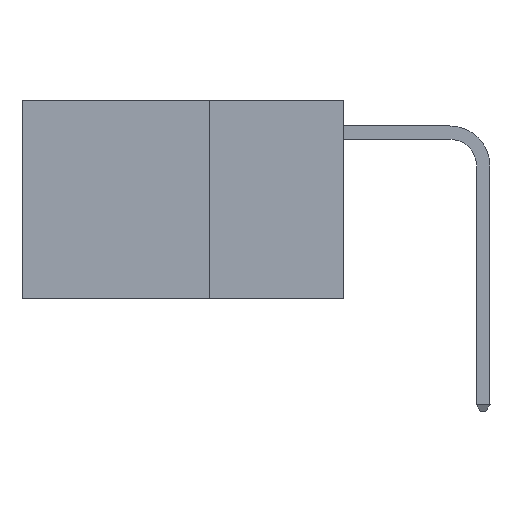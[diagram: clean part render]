
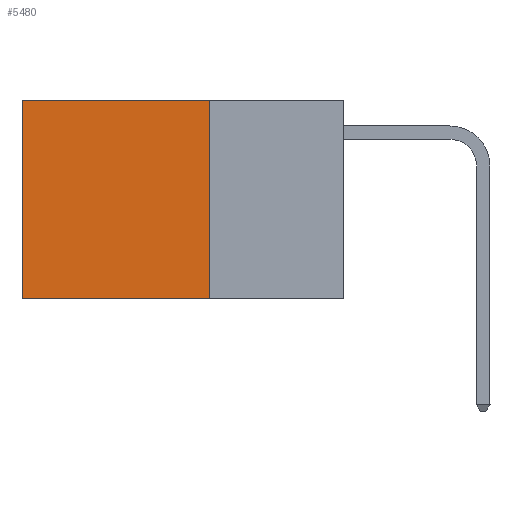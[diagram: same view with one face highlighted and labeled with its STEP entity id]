
A CAD part, left-side view. The second image highlights one B-rep face of the part: STEP entity #5480.
In plain terms, the highlighted planar face has unit normal (-1, 0, 0).
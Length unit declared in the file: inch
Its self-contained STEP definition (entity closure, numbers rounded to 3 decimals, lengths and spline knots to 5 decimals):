
#36 = DIRECTION ( 'NONE',  ( 0., 0., -1. ) ) ;
#154 = DIRECTION ( 'NONE',  ( 1., 0., 0. ) ) ;
#288 = CARTESIAN_POINT ( 'NONE',  ( 0.2625, 0.6, 0. ) ) ;
#402 = VERTEX_POINT ( 'NONE', #11299 ) ;
#487 = EDGE_CURVE ( 'NONE', #6970, #2752, #10767, .T. ) ;
#626 = ORIENTED_EDGE ( 'NONE', *, *, #5296, .F. ) ;
#1123 = ORIENTED_EDGE ( 'NONE', *, *, #6794, .F. ) ;
#2195 = CARTESIAN_POINT ( 'NONE',  ( 0.2625, 0.25, 0. ) ) ;
#2482 = CARTESIAN_POINT ( 'NONE',  ( 0.2625, 0.25, 0. ) ) ;
#2663 = FACE_OUTER_BOUND ( 'NONE', #4842, .T. ) ;
#2690 = VECTOR ( 'NONE', #9444, 39.37008 ) ;
#2752 = VERTEX_POINT ( 'NONE', #288 ) ;
#3452 = VECTOR ( 'NONE', #6245, 39.37008 ) ;
#3512 = AXIS2_PLACEMENT_3D ( 'NONE', #12744, #154, #7525 ) ;
#4135 = CARTESIAN_POINT ( 'NONE',  ( 0.2625, 0.6, 0. ) ) ;
#4176 = ORIENTED_EDGE ( 'NONE', *, *, #13438, .T. ) ;
#4400 = VERTEX_POINT ( 'NONE', #6271 ) ;
#4842 = EDGE_LOOP ( 'NONE', ( #4176, #626, #1123, #9926 ) ) ;
#5296 = EDGE_CURVE ( 'NONE', #402, #4400, #7436, .T. ) ;
#5407 = PLANE ( 'NONE',  #3512 ) ;
#5480 = ADVANCED_FACE ( 'NONE', ( #2663 ), #5407, .F. ) ;
#6245 = DIRECTION ( 'NONE',  ( 0., 0., -1. ) ) ;
#6271 = CARTESIAN_POINT ( 'NONE',  ( 0.2625, 0.6, -0.37 ) ) ;
#6794 = EDGE_CURVE ( 'NONE', #6970, #402, #7554, .T. ) ;
#6970 = VERTEX_POINT ( 'NONE', #2482 ) ;
#7436 = LINE ( 'NONE', #9280, #9919 ) ;
#7525 = DIRECTION ( 'NONE',  ( 0., 0., -1. ) ) ;
#7554 = LINE ( 'NONE', #2195, #10038 ) ;
#9280 = CARTESIAN_POINT ( 'NONE',  ( 0.2625, 0.25, -0.37 ) ) ;
#9444 = DIRECTION ( 'NONE',  ( 0., 1., 0. ) ) ;
#9480 = CARTESIAN_POINT ( 'NONE',  ( 0.2625, 0.25, 0. ) ) ;
#9919 = VECTOR ( 'NONE', #12426, 39.37008 ) ;
#9926 = ORIENTED_EDGE ( 'NONE', *, *, #487, .T. ) ;
#10038 = VECTOR ( 'NONE', #36, 39.37008 ) ;
#10767 = LINE ( 'NONE', #9480, #2690 ) ;
#11299 = CARTESIAN_POINT ( 'NONE',  ( 0.2625, 0.25, -0.37 ) ) ;
#11850 = LINE ( 'NONE', #4135, #3452 ) ;
#12426 = DIRECTION ( 'NONE',  ( 0., 1., 0. ) ) ;
#12744 = CARTESIAN_POINT ( 'NONE',  ( 0.2625, 0.25, 0. ) ) ;
#13438 = EDGE_CURVE ( 'NONE', #2752, #4400, #11850, .T. ) ;
